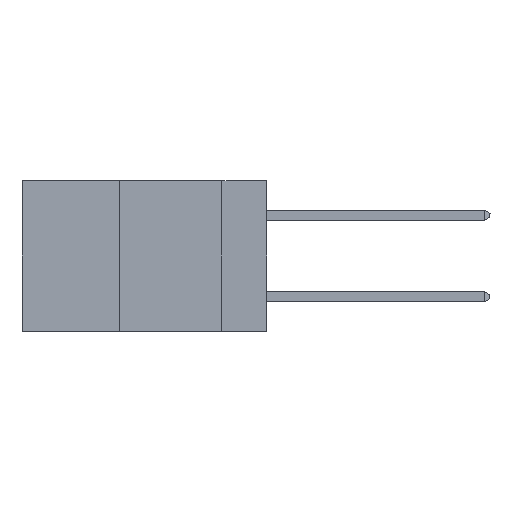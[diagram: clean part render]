
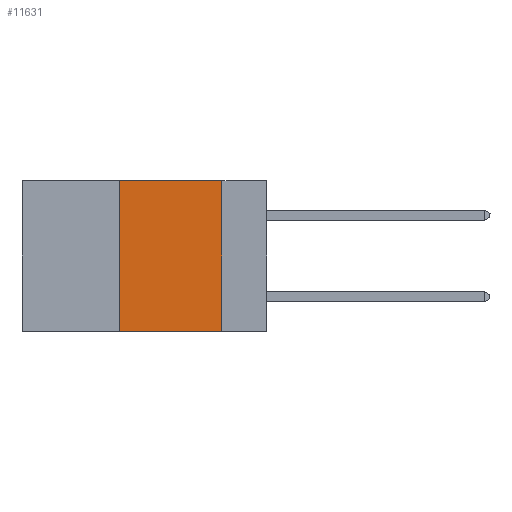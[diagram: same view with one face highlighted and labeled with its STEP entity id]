
A CAD part, left-side view. The second image highlights one B-rep face of the part: STEP entity #11631.
In plain terms, the highlighted planar face has unit normal (-1, 0, 0).
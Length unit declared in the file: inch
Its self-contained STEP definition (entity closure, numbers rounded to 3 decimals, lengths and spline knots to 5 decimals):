
#323 = VECTOR ( 'NONE', #4292, 39.37008 ) ;
#2025 = DIRECTION ( 'NONE',  ( 0., 0., 1. ) ) ;
#2218 = EDGE_CURVE ( 'NONE', #17064, #15416, #6184, .T. ) ;
#2617 = DIRECTION ( 'NONE',  ( 0., 0., -1. ) ) ;
#2934 = CARTESIAN_POINT ( 'NONE',  ( 0., 0.6, -0.37 ) ) ;
#3165 = VECTOR ( 'NONE', #9292, 39.37008 ) ;
#3512 = DIRECTION ( 'NONE',  ( 0., 0., -1. ) ) ;
#3644 = CARTESIAN_POINT ( 'NONE',  ( 0., 0.36, 0. ) ) ;
#3781 = CARTESIAN_POINT ( 'NONE',  ( 0., 0.36, -0.37 ) ) ;
#4292 = DIRECTION ( 'NONE',  ( 0., -1., 0. ) ) ;
#5554 = ORIENTED_EDGE ( 'NONE', *, *, #16144, .F. ) ;
#5630 = CARTESIAN_POINT ( 'NONE',  ( 0., 0.11, 0. ) ) ;
#6184 = LINE ( 'NONE', #10777, #3165 ) ;
#6847 = LINE ( 'NONE', #2934, #323 ) ;
#7592 = VECTOR ( 'NONE', #2025, 39.37008 ) ;
#8036 = LINE ( 'NONE', #15275, #7592 ) ;
#8332 = EDGE_CURVE ( 'NONE', #13563, #18256, #6847, .T. ) ;
#9292 = DIRECTION ( 'NONE',  ( 0., -1., 0. ) ) ;
#9356 = CARTESIAN_POINT ( 'NONE',  ( 0., 0.6, 0. ) ) ;
#9806 = ORIENTED_EDGE ( 'NONE', *, *, #2218, .F. ) ;
#10777 = CARTESIAN_POINT ( 'NONE',  ( 0., 0.6, 0. ) ) ;
#10927 = FACE_OUTER_BOUND ( 'NONE', #14419, .T. ) ;
#11166 = CARTESIAN_POINT ( 'NONE',  ( 0., 0.11, 0. ) ) ;
#11631 = ADVANCED_FACE ( 'NONE', ( #10927 ), #12471, .F. ) ;
#11851 = ORIENTED_EDGE ( 'NONE', *, *, #15206, .F. ) ;
#12471 = PLANE ( 'NONE',  #18136 ) ;
#13563 = VERTEX_POINT ( 'NONE', #3781 ) ;
#13857 = VECTOR ( 'NONE', #2617, 39.37008 ) ;
#14419 = EDGE_LOOP ( 'NONE', ( #5554, #9806, #11851, #16333 ) ) ;
#15206 = EDGE_CURVE ( 'NONE', #13563, #17064, #8036, .T. ) ;
#15275 = CARTESIAN_POINT ( 'NONE',  ( 0., 0.36, 0. ) ) ;
#15416 = VERTEX_POINT ( 'NONE', #11166 ) ;
#15686 = DIRECTION ( 'NONE',  ( 1., 0., 0. ) ) ;
#16144 = EDGE_CURVE ( 'NONE', #15416, #18256, #17611, .T. ) ;
#16333 = ORIENTED_EDGE ( 'NONE', *, *, #8332, .T. ) ;
#17064 = VERTEX_POINT ( 'NONE', #3644 ) ;
#17611 = LINE ( 'NONE', #5630, #13857 ) ;
#18136 = AXIS2_PLACEMENT_3D ( 'NONE', #9356, #15686, #3512 ) ;
#18256 = VERTEX_POINT ( 'NONE', #18265 ) ;
#18265 = CARTESIAN_POINT ( 'NONE',  ( 0., 0.11, -0.37 ) ) ;
